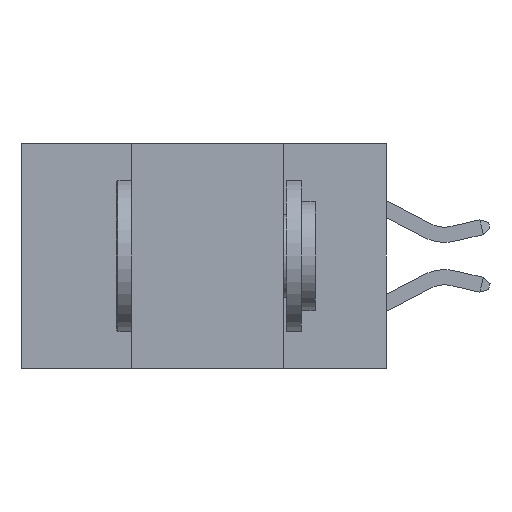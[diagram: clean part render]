
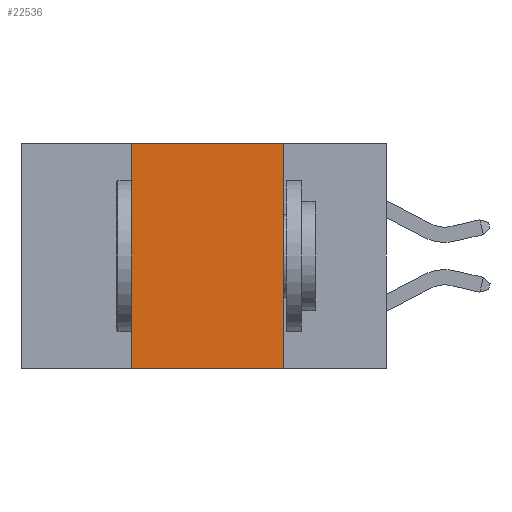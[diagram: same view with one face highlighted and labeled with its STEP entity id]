
A CAD part, left-side view. The second image highlights one B-rep face of the part: STEP entity #22536.
In plain terms, the highlighted planar face has unit normal (-1, 0, 0).
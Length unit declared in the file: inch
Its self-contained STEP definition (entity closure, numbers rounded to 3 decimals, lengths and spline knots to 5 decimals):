
#765 = CARTESIAN_POINT ( 'NONE',  ( 0., 0.17, 0. ) ) ;
#814 = DIRECTION ( 'NONE',  ( 0., 0., -1. ) ) ;
#1057 = CARTESIAN_POINT ( 'NONE',  ( 0., 0.6, 0. ) ) ;
#1202 = LINE ( 'NONE', #22634, #18019 ) ;
#1234 = CARTESIAN_POINT ( 'NONE',  ( 0., 0.17, -0.37 ) ) ;
#3760 = AXIS2_PLACEMENT_3D ( 'NONE', #19373, #6779, #21430 ) ;
#4250 = EDGE_CURVE ( 'NONE', #5440, #12418, #1202, .T. ) ;
#4651 = PLANE ( 'NONE',  #3760 ) ;
#5218 = LINE ( 'NONE', #1057, #15788 ) ;
#5440 = VERTEX_POINT ( 'NONE', #26537 ) ;
#5682 = EDGE_CURVE ( 'NONE', #5440, #9643, #11034, .T. ) ;
#6779 = DIRECTION ( 'NONE',  ( 1., 0., 0. ) ) ;
#9134 = ORIENTED_EDGE ( 'NONE', *, *, #20118, .F. ) ;
#9643 = VERTEX_POINT ( 'NONE', #19557 ) ;
#9801 = ORIENTED_EDGE ( 'NONE', *, *, #24720, .F. ) ;
#11034 = LINE ( 'NONE', #20083, #11703 ) ;
#11243 = CARTESIAN_POINT ( 'NONE',  ( 0., 0.17, -0.37 ) ) ;
#11703 = VECTOR ( 'NONE', #22940, 39.37008 ) ;
#12418 = VERTEX_POINT ( 'NONE', #1234 ) ;
#14024 = VECTOR ( 'NONE', #814, 39.37008 ) ;
#14230 = FACE_OUTER_BOUND ( 'NONE', #22827, .T. ) ;
#15788 = VECTOR ( 'NONE', #26151, 39.37008 ) ;
#18019 = VECTOR ( 'NONE', #24694, 39.37008 ) ;
#19373 = CARTESIAN_POINT ( 'NONE',  ( 0., 0.6, 0. ) ) ;
#19557 = CARTESIAN_POINT ( 'NONE',  ( 0., 0.42, 0. ) ) ;
#20083 = CARTESIAN_POINT ( 'NONE',  ( 0., 0.42, -0.37 ) ) ;
#20118 = EDGE_CURVE ( 'NONE', #25332, #12418, #26306, .T. ) ;
#20914 = ORIENTED_EDGE ( 'NONE', *, *, #5682, .F. ) ;
#21430 = DIRECTION ( 'NONE',  ( 0., 0., -1. ) ) ;
#21548 = ORIENTED_EDGE ( 'NONE', *, *, #4250, .T. ) ;
#22536 = ADVANCED_FACE ( 'NONE', ( #14230 ), #4651, .F. ) ;
#22634 = CARTESIAN_POINT ( 'NONE',  ( 0., 0.6, -0.37 ) ) ;
#22827 = EDGE_LOOP ( 'NONE', ( #9134, #9801, #20914, #21548 ) ) ;
#22940 = DIRECTION ( 'NONE',  ( 0., 0., 1. ) ) ;
#24694 = DIRECTION ( 'NONE',  ( 0., -1., 0. ) ) ;
#24720 = EDGE_CURVE ( 'NONE', #9643, #25332, #5218, .T. ) ;
#25332 = VERTEX_POINT ( 'NONE', #765 ) ;
#26151 = DIRECTION ( 'NONE',  ( 0., -1., 0. ) ) ;
#26306 = LINE ( 'NONE', #11243, #14024 ) ;
#26537 = CARTESIAN_POINT ( 'NONE',  ( 0., 0.42, -0.37 ) ) ;
